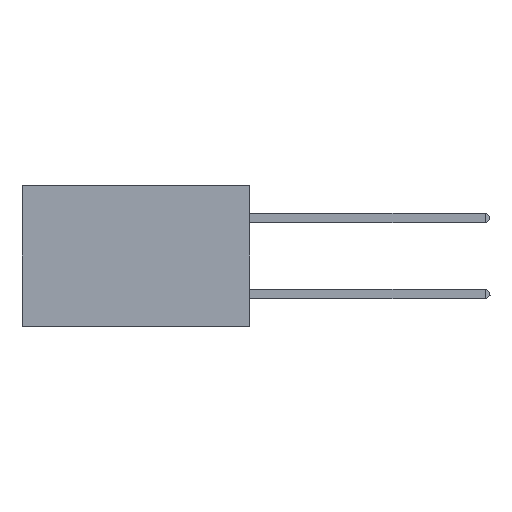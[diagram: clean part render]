
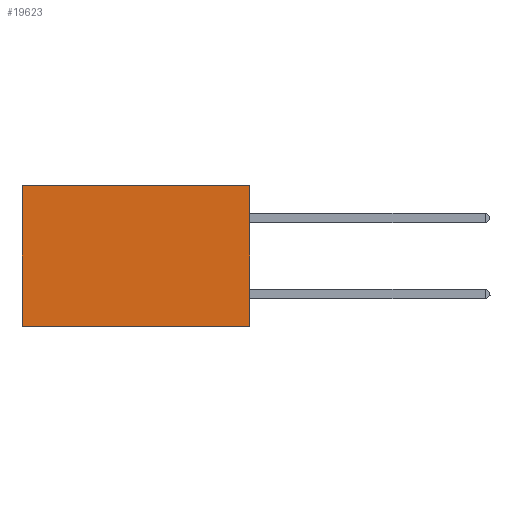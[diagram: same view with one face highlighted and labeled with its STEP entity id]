
A CAD part, left-side view. The second image highlights one B-rep face of the part: STEP entity #19623.
In plain terms, the highlighted planar face has unit normal (-1, 0, 0).
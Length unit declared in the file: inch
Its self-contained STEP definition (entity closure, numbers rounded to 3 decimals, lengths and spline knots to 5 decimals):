
#1915 = FACE_OUTER_BOUND ( 'NONE', #7921, .T. ) ;
#2157 = CARTESIAN_POINT ( 'NONE',  ( 0.2875, 0., -0.37 ) ) ;
#3561 = DIRECTION ( 'NONE',  ( 1., 0., 0. ) ) ;
#3765 = DIRECTION ( 'NONE',  ( 0., 0., -1. ) ) ;
#4891 = LINE ( 'NONE', #28370, #16205 ) ;
#4895 = VERTEX_POINT ( 'NONE', #41817 ) ;
#6526 = CARTESIAN_POINT ( 'NONE',  ( 0.2875, 0.6, 0. ) ) ;
#6862 = PLANE ( 'NONE',  #22559 ) ;
#7817 = ORIENTED_EDGE ( 'NONE', *, *, #40333, .F. ) ;
#7921 = EDGE_LOOP ( 'NONE', ( #41297, #40753, #7817, #33160 ) ) ;
#8015 = CARTESIAN_POINT ( 'NONE',  ( 0.2875, 0.6, 0. ) ) ;
#9186 = VECTOR ( 'NONE', #37251, 39.37008 ) ;
#10230 = LINE ( 'NONE', #35079, #9186 ) ;
#14204 = VERTEX_POINT ( 'NONE', #6526 ) ;
#16205 = VECTOR ( 'NONE', #24788, 39.37008 ) ;
#18447 = EDGE_CURVE ( 'NONE', #14204, #4895, #39960, .T. ) ;
#19623 = ADVANCED_FACE ( 'NONE', ( #1915 ), #6862, .F. ) ;
#20095 = LINE ( 'NONE', #27276, #25729 ) ;
#22522 = VECTOR ( 'NONE', #30957, 39.37008 ) ;
#22559 = AXIS2_PLACEMENT_3D ( 'NONE', #35962, #3561, #39120 ) ;
#23023 = EDGE_CURVE ( 'NONE', #31738, #4895, #4891, .T. ) ;
#24788 = DIRECTION ( 'NONE',  ( 0., 1., 0. ) ) ;
#25729 = VECTOR ( 'NONE', #3765, 39.37008 ) ;
#27237 = EDGE_CURVE ( 'NONE', #33855, #14204, #10230, .T. ) ;
#27276 = CARTESIAN_POINT ( 'NONE',  ( 0.2875, 0., 0. ) ) ;
#28370 = CARTESIAN_POINT ( 'NONE',  ( 0.2875, 0., -0.37 ) ) ;
#29700 = CARTESIAN_POINT ( 'NONE',  ( 0.2875, 0., 0. ) ) ;
#30957 = DIRECTION ( 'NONE',  ( 0., 0., -1. ) ) ;
#31738 = VERTEX_POINT ( 'NONE', #2157 ) ;
#33160 = ORIENTED_EDGE ( 'NONE', *, *, #27237, .T. ) ;
#33855 = VERTEX_POINT ( 'NONE', #29700 ) ;
#35079 = CARTESIAN_POINT ( 'NONE',  ( 0.2875, 0., 0. ) ) ;
#35962 = CARTESIAN_POINT ( 'NONE',  ( 0.2875, 0., 0. ) ) ;
#37251 = DIRECTION ( 'NONE',  ( 0., 1., 0. ) ) ;
#39120 = DIRECTION ( 'NONE',  ( 0., 0., -1. ) ) ;
#39960 = LINE ( 'NONE', #8015, #22522 ) ;
#40333 = EDGE_CURVE ( 'NONE', #33855, #31738, #20095, .T. ) ;
#40753 = ORIENTED_EDGE ( 'NONE', *, *, #23023, .F. ) ;
#41297 = ORIENTED_EDGE ( 'NONE', *, *, #18447, .T. ) ;
#41817 = CARTESIAN_POINT ( 'NONE',  ( 0.2875, 0.6, -0.37 ) ) ;
